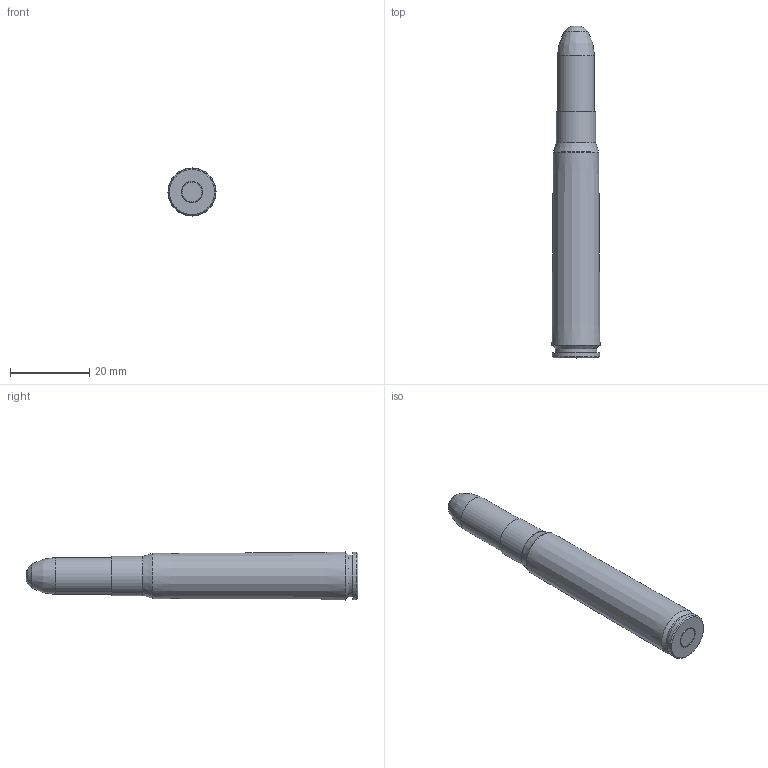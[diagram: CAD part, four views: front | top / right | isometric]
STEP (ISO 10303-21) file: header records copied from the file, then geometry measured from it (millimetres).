
FILE_DESCRIPTION((''),'2;1');
FILE_NAME('9.2X62MM MAUSER.stp','2012-12-05T13:31:04',('AGARRETT'),(''),'Autodesk Inventor 2012','Autodesk Inventor 2012','');
FILE_SCHEMA(('AUTOMOTIVE_DESIGN { 1 0 10303 214 1 1 1 1 }'));
Length unit declared in the file: inch
Products named in the file (4): iLogic Cartridge; Rimless Bottleneck; iLogic RN Bullet; PRIMER
Assembly tree (3 placements, depth 2):
  iLogic Cartridge
    Rimless Bottleneck
    iLogic RN Bullet
    PRIMER
Bounding box: 12.1 x 83.6 x 12.1 mm (x, y, z)
Volume: 2897 mm3; surface area: 5617.9 mm2
Topology: 3 solids, 3 shells, 35 faces, 59 edges, 33 vertices
Faces by surface type: plane 9, cylinder 9, torus 8, cone 7, bspline 2
Full cylindrical faces by diameter (mm): 1.778 x1, 5.08 x1, 5.334 x2, 9.299 x2, 9.921 x1, 10.5 x1, 11.951 x1
Entity records: 878 total; most frequent: CARTESIAN_POINT 160, DIRECTION 146, AXIS2_PLACEMENT_3D 73, ORIENTED_EDGE 66, EDGE_LOOP 66, FACE_OUTER_BOUND 35, ADVANCED_FACE 35, VERTEX_POINT 33
